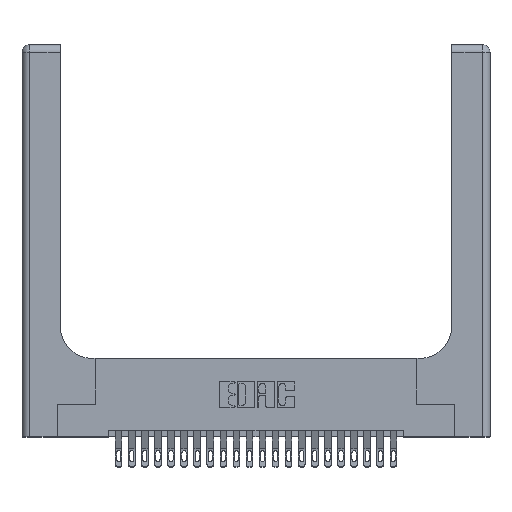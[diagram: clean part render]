
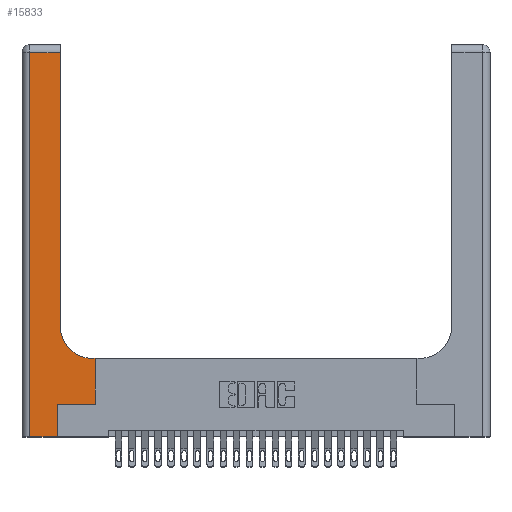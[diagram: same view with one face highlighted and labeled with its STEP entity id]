
A CAD part, top view. The second image highlights one B-rep face of the part: STEP entity #15833.
In plain terms, the highlighted planar face has unit normal (0, 0, 1).
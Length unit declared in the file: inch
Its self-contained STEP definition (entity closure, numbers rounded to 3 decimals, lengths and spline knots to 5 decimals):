
#70 = ORIENTED_EDGE ( 'NONE', *, *, #11249, .T. ) ;
#178 = CARTESIAN_POINT ( 'NONE',  ( 0.2915, 3., 0.37 ) ) ;
#501 = DIRECTION ( 'NONE',  ( -1., 0., 0. ) ) ;
#524 = EDGE_CURVE ( 'NONE', #13312, #5602, #22209, .T. ) ;
#772 = LINE ( 'NONE', #24919, #10840 ) ;
#1416 = DIRECTION ( 'NONE',  ( 0., -1., 0. ) ) ;
#2249 = CARTESIAN_POINT ( 'NONE',  ( 0., 0., 0.37 ) ) ;
#2307 = LINE ( 'NONE', #19279, #6959 ) ;
#2582 = CARTESIAN_POINT ( 'NONE',  ( 0., 2.94, 0.37 ) ) ;
#2638 = ORIENTED_EDGE ( 'NONE', *, *, #12640, .T. ) ;
#3146 = VERTEX_POINT ( 'NONE', #9016 ) ;
#3277 = VECTOR ( 'NONE', #22038, 39.37008 ) ;
#3446 = CARTESIAN_POINT ( 'NONE',  ( 0.2915, 0.85, 0.37 ) ) ;
#3962 = EDGE_CURVE ( 'NONE', #3146, #20289, #2307, .T. ) ;
#4285 = LINE ( 'NONE', #9714, #14246 ) ;
#4689 = VERTEX_POINT ( 'NONE', #23599 ) ;
#4694 = LINE ( 'NONE', #23188, #24873 ) ;
#5602 = VERTEX_POINT ( 'NONE', #12571 ) ;
#6778 = ORIENTED_EDGE ( 'NONE', *, *, #14591, .T. ) ;
#6959 = VECTOR ( 'NONE', #15370, 39.37008 ) ;
#7455 = AXIS2_PLACEMENT_3D ( 'NONE', #8282, #22013, #10331 ) ;
#8282 = CARTESIAN_POINT ( 'NONE',  ( 0.5415, 0.85, 0.37 ) ) ;
#9016 = CARTESIAN_POINT ( 'NONE',  ( 0.5585, 0.6, 0.37 ) ) ;
#9070 = ORIENTED_EDGE ( 'NONE', *, *, #24249, .T. ) ;
#9556 = DIRECTION ( 'NONE',  ( 1., 0., 0. ) ) ;
#9714 = CARTESIAN_POINT ( 'NONE',  ( 0.5585, 0.25, 0.37 ) ) ;
#9966 = CIRCLE ( 'NONE', #7455, 0.25 ) ;
#10331 = DIRECTION ( 'NONE',  ( 1., 0., 0. ) ) ;
#10357 = CARTESIAN_POINT ( 'NONE',  ( 0.269, 0., 0.37 ) ) ;
#10603 = DIRECTION ( 'NONE',  ( 0., 0., -1. ) ) ;
#10611 = ORIENTED_EDGE ( 'NONE', *, *, #11575, .T. ) ;
#10746 = VECTOR ( 'NONE', #12293, 39.37008 ) ;
#10840 = VECTOR ( 'NONE', #1416, 39.37008 ) ;
#10859 = ORIENTED_EDGE ( 'NONE', *, *, #3962, .T. ) ;
#11163 = ORIENTED_EDGE ( 'NONE', *, *, #24474, .T. ) ;
#11167 = EDGE_CURVE ( 'NONE', #11966, #17230, #23512, .T. ) ;
#11249 = EDGE_CURVE ( 'NONE', #5602, #15789, #21738, .T. ) ;
#11338 = CARTESIAN_POINT ( 'NONE',  ( 0.5585, 0.25, 0.37 ) ) ;
#11575 = EDGE_CURVE ( 'NONE', #19158, #3146, #4285, .T. ) ;
#11860 = VECTOR ( 'NONE', #22545, 39.37008 ) ;
#11966 = VERTEX_POINT ( 'NONE', #14878 ) ;
#12293 = DIRECTION ( 'NONE',  ( 1., 0., 0. ) ) ;
#12525 = FACE_OUTER_BOUND ( 'NONE', #16620, .T. ) ;
#12571 = CARTESIAN_POINT ( 'NONE',  ( 0.2915, 2.94, 0.37 ) ) ;
#12640 = EDGE_CURVE ( 'NONE', #15789, #4689, #772, .T. ) ;
#13312 = VERTEX_POINT ( 'NONE', #3446 ) ;
#14246 = VECTOR ( 'NONE', #21417, 39.37008 ) ;
#14304 = ORIENTED_EDGE ( 'NONE', *, *, #524, .T. ) ;
#14393 = CARTESIAN_POINT ( 'NONE',  ( 0.06, 2.94, 0.37 ) ) ;
#14591 = EDGE_CURVE ( 'NONE', #4689, #11966, #21113, .T. ) ;
#14878 = CARTESIAN_POINT ( 'NONE',  ( 0.269, 0., 0.37 ) ) ;
#15370 = DIRECTION ( 'NONE',  ( -1., 0., 0. ) ) ;
#15789 = VERTEX_POINT ( 'NONE', #14393 ) ;
#15833 = ADVANCED_FACE ( 'NONE', ( #12525 ), #22269, .F. ) ;
#16620 = EDGE_LOOP ( 'NONE', ( #14304, #70, #2638, #6778, #20340, #9070, #10611, #10859, #11163 ) ) ;
#16795 = CARTESIAN_POINT ( 'NONE',  ( 0.269, 0.25, 0.37 ) ) ;
#17201 = VECTOR ( 'NONE', #501, 39.37008 ) ;
#17230 = VERTEX_POINT ( 'NONE', #16795 ) ;
#17452 = CARTESIAN_POINT ( 'NONE',  ( 0.5415, 0.6, 0.37 ) ) ;
#18388 = CARTESIAN_POINT ( 'NONE',  ( 0., 3., 0.37 ) ) ;
#19158 = VERTEX_POINT ( 'NONE', #11338 ) ;
#19279 = CARTESIAN_POINT ( 'NONE',  ( 0.2915, 0.6, 0.37 ) ) ;
#20289 = VERTEX_POINT ( 'NONE', #17452 ) ;
#20340 = ORIENTED_EDGE ( 'NONE', *, *, #11167, .T. ) ;
#21113 = LINE ( 'NONE', #2249, #10746 ) ;
#21417 = DIRECTION ( 'NONE',  ( 0., 1., 0. ) ) ;
#21738 = LINE ( 'NONE', #2582, #17201 ) ;
#22013 = DIRECTION ( 'NONE',  ( 0., 0., -1. ) ) ;
#22038 = DIRECTION ( 'NONE',  ( 0., 1., 0. ) ) ;
#22209 = LINE ( 'NONE', #178, #11860 ) ;
#22269 = PLANE ( 'NONE',  #24978 ) ;
#22545 = DIRECTION ( 'NONE',  ( 0., 1., 0. ) ) ;
#23188 = CARTESIAN_POINT ( 'NONE',  ( 0.269, 0.25, 0.37 ) ) ;
#23512 = LINE ( 'NONE', #10357, #3277 ) ;
#23599 = CARTESIAN_POINT ( 'NONE',  ( 0.06, 0., 0.37 ) ) ;
#24150 = DIRECTION ( 'NONE',  ( -1., 0., 0. ) ) ;
#24249 = EDGE_CURVE ( 'NONE', #17230, #19158, #4694, .T. ) ;
#24474 = EDGE_CURVE ( 'NONE', #20289, #13312, #9966, .T. ) ;
#24873 = VECTOR ( 'NONE', #9556, 39.37008 ) ;
#24919 = CARTESIAN_POINT ( 'NONE',  ( 0.06, 3., 0.37 ) ) ;
#24978 = AXIS2_PLACEMENT_3D ( 'NONE', #18388, #10603, #24150 ) ;
